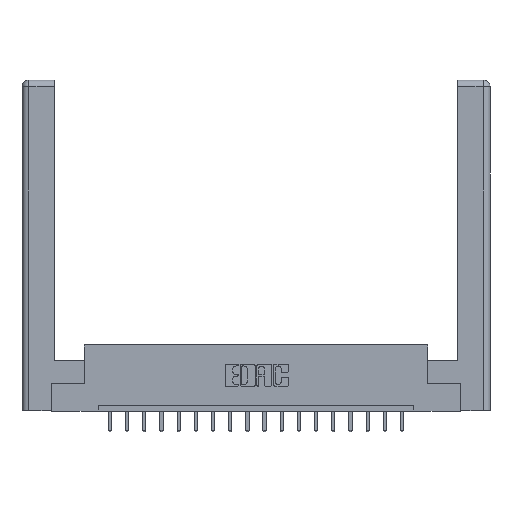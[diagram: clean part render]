
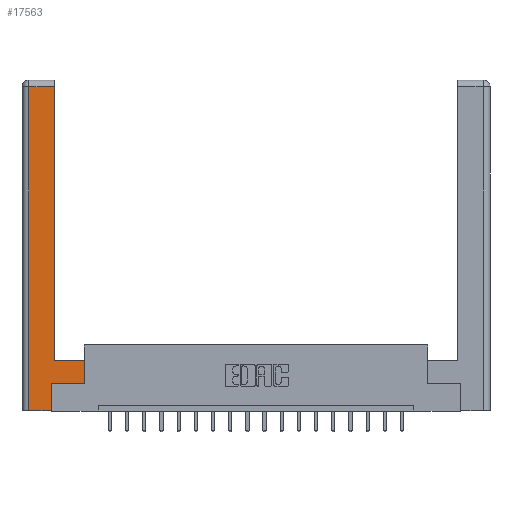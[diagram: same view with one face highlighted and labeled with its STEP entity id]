
A CAD part, top view. The second image highlights one B-rep face of the part: STEP entity #17563.
In plain terms, the highlighted planar face has unit normal (0, 0, 1).
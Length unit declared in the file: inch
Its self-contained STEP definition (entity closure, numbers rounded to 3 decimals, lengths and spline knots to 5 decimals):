
#37 = DIRECTION ( 'NONE',  ( 0., 1., 0. ) ) ;
#218 = CARTESIAN_POINT ( 'NONE',  ( 0.0615, 2.94, 0. ) ) ;
#332 = CARTESIAN_POINT ( 'NONE',  ( 0.565, 0.245, 0. ) ) ;
#361 = EDGE_CURVE ( 'NONE', #3939, #13530, #4235, .T. ) ;
#784 = DIRECTION ( 'NONE',  ( 0., -1., 0. ) ) ;
#1009 = DIRECTION ( 'NONE',  ( 1., 0., 0. ) ) ;
#1022 = CARTESIAN_POINT ( 'NONE',  ( 0.565, 0.45, 0. ) ) ;
#1408 = VERTEX_POINT ( 'NONE', #2241 ) ;
#1642 = VECTOR ( 'NONE', #14616, 39.37008 ) ;
#1945 = EDGE_CURVE ( 'NONE', #12428, #12131, #18161, .T. ) ;
#2241 = CARTESIAN_POINT ( 'NONE',  ( 0.265, 0.245, 0. ) ) ;
#2746 = PLANE ( 'NONE',  #5178 ) ;
#3236 = DIRECTION ( 'NONE',  ( -1., 0., 0. ) ) ;
#3280 = EDGE_CURVE ( 'NONE', #13530, #15319, #14414, .T. ) ;
#3830 = EDGE_CURVE ( 'NONE', #1408, #3939, #16038, .T. ) ;
#3939 = VERTEX_POINT ( 'NONE', #9417 ) ;
#4014 = EDGE_CURVE ( 'NONE', #15319, #18628, #10249, .T. ) ;
#4235 = LINE ( 'NONE', #10613, #13107 ) ;
#4303 = EDGE_LOOP ( 'NONE', ( #12618, #11073, #7091, #8673, #10697, #14497, #9846, #9039 ) ) ;
#4512 = DIRECTION ( 'NONE',  ( 0., 0., -1. ) ) ;
#4680 = VERTEX_POINT ( 'NONE', #218 ) ;
#4909 = LINE ( 'NONE', #5066, #8436 ) ;
#5066 = CARTESIAN_POINT ( 'NONE',  ( 0.0615, 0., 0. ) ) ;
#5178 = AXIS2_PLACEMENT_3D ( 'NONE', #10476, #4512, #8718 ) ;
#5402 = EDGE_CURVE ( 'NONE', #12131, #1408, #5726, .T. ) ;
#5726 = LINE ( 'NONE', #17580, #7359 ) ;
#5990 = VECTOR ( 'NONE', #15653, 39.37008 ) ;
#6271 = VECTOR ( 'NONE', #1009, 39.37008 ) ;
#6683 = VECTOR ( 'NONE', #16926, 39.37008 ) ;
#7091 = ORIENTED_EDGE ( 'NONE', *, *, #15891, .T. ) ;
#7359 = VECTOR ( 'NONE', #17636, 39.37008 ) ;
#7878 = FACE_OUTER_BOUND ( 'NONE', #4303, .T. ) ;
#8436 = VECTOR ( 'NONE', #784, 39.37008 ) ;
#8673 = ORIENTED_EDGE ( 'NONE', *, *, #1945, .T. ) ;
#8718 = DIRECTION ( 'NONE',  ( -1., 0., 0. ) ) ;
#9039 = ORIENTED_EDGE ( 'NONE', *, *, #3280, .T. ) ;
#9417 = CARTESIAN_POINT ( 'NONE',  ( 0.565, 0.245, 0. ) ) ;
#9846 = ORIENTED_EDGE ( 'NONE', *, *, #361, .T. ) ;
#9847 = CARTESIAN_POINT ( 'NONE',  ( 0.265, 0., 0. ) ) ;
#10004 = VECTOR ( 'NONE', #3236, 39.37008 ) ;
#10249 = LINE ( 'NONE', #15769, #5990 ) ;
#10476 = CARTESIAN_POINT ( 'NONE',  ( 0., 0., 0. ) ) ;
#10613 = CARTESIAN_POINT ( 'NONE',  ( 0.565, 0.45, 0. ) ) ;
#10697 = ORIENTED_EDGE ( 'NONE', *, *, #5402, .T. ) ;
#11073 = ORIENTED_EDGE ( 'NONE', *, *, #12025, .T. ) ;
#11131 = CARTESIAN_POINT ( 'NONE',  ( 0.0615, 0., 0. ) ) ;
#12025 = EDGE_CURVE ( 'NONE', #18628, #4680, #14243, .T. ) ;
#12131 = VERTEX_POINT ( 'NONE', #16140 ) ;
#12428 = VERTEX_POINT ( 'NONE', #11131 ) ;
#12618 = ORIENTED_EDGE ( 'NONE', *, *, #4014, .T. ) ;
#13107 = VECTOR ( 'NONE', #37, 39.37008 ) ;
#13296 = CARTESIAN_POINT ( 'NONE',  ( 0.0615, 2.94, 0. ) ) ;
#13530 = VERTEX_POINT ( 'NONE', #1022 ) ;
#14243 = LINE ( 'NONE', #13296, #1642 ) ;
#14414 = LINE ( 'NONE', #18092, #10004 ) ;
#14497 = ORIENTED_EDGE ( 'NONE', *, *, #3830, .T. ) ;
#14521 = CARTESIAN_POINT ( 'NONE',  ( 0.295, 0.45, 0. ) ) ;
#14616 = DIRECTION ( 'NONE',  ( -1., 0., 0. ) ) ;
#15319 = VERTEX_POINT ( 'NONE', #14521 ) ;
#15653 = DIRECTION ( 'NONE',  ( 0., 1., 0. ) ) ;
#15769 = CARTESIAN_POINT ( 'NONE',  ( 0.295, 3., 0. ) ) ;
#15891 = EDGE_CURVE ( 'NONE', #4680, #12428, #4909, .T. ) ;
#16038 = LINE ( 'NONE', #332, #6683 ) ;
#16140 = CARTESIAN_POINT ( 'NONE',  ( 0.265, 0., 0. ) ) ;
#16926 = DIRECTION ( 'NONE',  ( 1., 0., 0. ) ) ;
#17202 = CARTESIAN_POINT ( 'NONE',  ( 0.295, 2.94, 0. ) ) ;
#17563 = ADVANCED_FACE ( 'NONE', ( #7878 ), #2746, .F. ) ;
#17580 = CARTESIAN_POINT ( 'NONE',  ( 0.265, 0.245, 0. ) ) ;
#17636 = DIRECTION ( 'NONE',  ( 0., 1., 0. ) ) ;
#18092 = CARTESIAN_POINT ( 'NONE',  ( 0.295, 0.45, 0. ) ) ;
#18161 = LINE ( 'NONE', #9847, #6271 ) ;
#18628 = VERTEX_POINT ( 'NONE', #17202 ) ;
